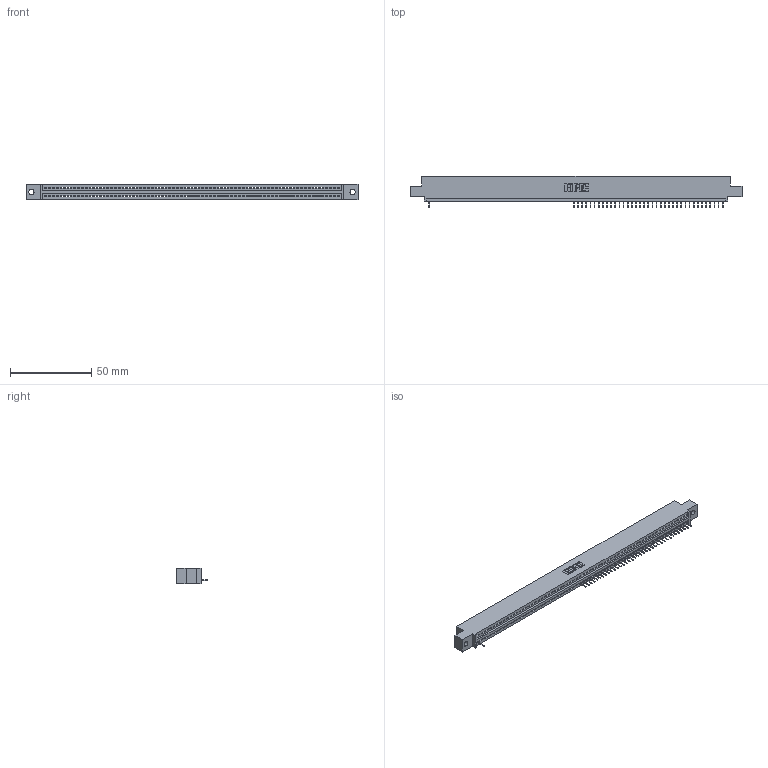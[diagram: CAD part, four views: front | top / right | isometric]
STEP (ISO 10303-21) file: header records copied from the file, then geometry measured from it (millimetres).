
FILE_DESCRIPTION (( 'STEP AP203' ), '1' );
FILE_NAME ('395-072-524-402.STEP', '2018-11-27T10:18:22', ( '' ), ( '' ), 'SwSTEP 2.0', 'SolidWorks 2016', '' );
FILE_SCHEMA (( 'CONFIG_CONTROL_DESIGN' ));
Length unit declared in the file: inch
Products named in the file (3): 395-072-524-402; 345 Part_0.110 Offset - 0.128 Dia; 345-292-001_345-293-124
Assembly tree (39 placements, depth 2):
  395-072-524-402
    345 Part_0.110 Offset - 0.128 Dia
    345-292-001_345-293-124  x38
Bounding box: 204.09 x 19.35 x 9.4 mm (x, y, z)
Volume: 18980.8 mm3; surface area: 22894.4 mm2
Topology: 39 solids, 39 shells, 3030 faces, 9029 edges, 5866 vertices
Faces by surface type: plane 2308, cylinder 722
Entity records: 49271 total; most frequent: ORIENTED_EDGE 8734, CARTESIAN_POINT 8694, DIRECTION 7511, EDGE_CURVE 4367, LINE 3951, VECTOR 3951, VERTEX_POINT 2906, AXIS2_PLACEMENT_3D 1780
